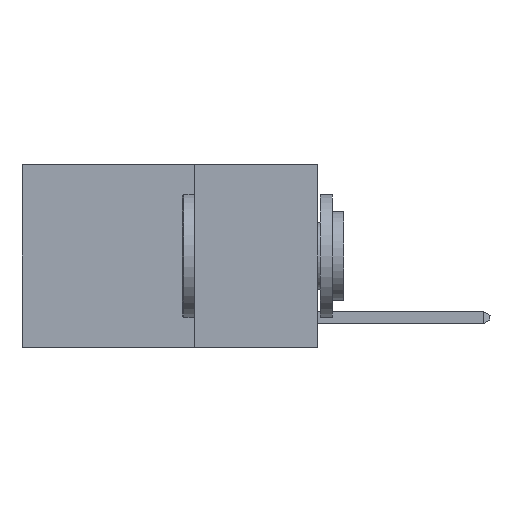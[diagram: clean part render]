
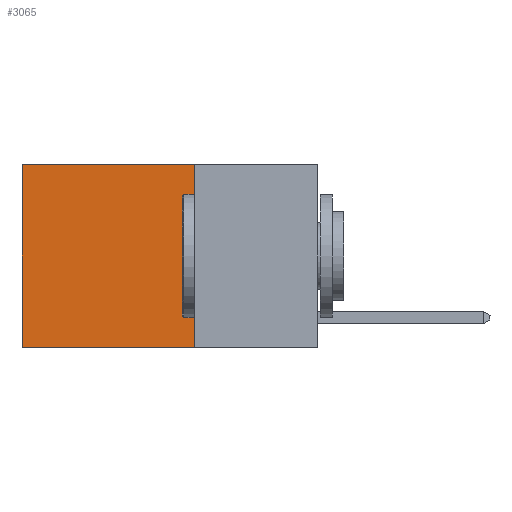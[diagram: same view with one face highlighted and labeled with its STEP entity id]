
A CAD part, left-side view. The second image highlights one B-rep face of the part: STEP entity #3065.
In plain terms, the highlighted planar face has unit normal (-1, 0, 0).
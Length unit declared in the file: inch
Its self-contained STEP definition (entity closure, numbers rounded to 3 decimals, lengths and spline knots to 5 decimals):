
#379 = LINE ( 'NONE', #10572, #13702 ) ;
#809 = CARTESIAN_POINT ( 'NONE',  ( 0.2625, 0.25, 0. ) ) ;
#1155 = LINE ( 'NONE', #1375, #1506 ) ;
#1322 = CARTESIAN_POINT ( 'NONE',  ( 0.2625, 0.6, -0.37 ) ) ;
#1352 = CARTESIAN_POINT ( 'NONE',  ( 0.2625, 0.6, 0. ) ) ;
#1375 = CARTESIAN_POINT ( 'NONE',  ( 0.2625, 0.25, 0. ) ) ;
#1506 = VECTOR ( 'NONE', #14447, 39.37008 ) ;
#1515 = DIRECTION ( 'NONE',  ( 1., 0., 0. ) ) ;
#1536 = EDGE_CURVE ( 'NONE', #3499, #5440, #1155, .T. ) ;
#2265 = EDGE_LOOP ( 'NONE', ( #4382, #9099, #7632, #3853 ) ) ;
#2464 = DIRECTION ( 'NONE',  ( 0., 0., -1. ) ) ;
#3065 = ADVANCED_FACE ( 'NONE', ( #7215 ), #10969, .F. ) ;
#3499 = VERTEX_POINT ( 'NONE', #809 ) ;
#3853 = ORIENTED_EDGE ( 'NONE', *, *, #1536, .T. ) ;
#4382 = ORIENTED_EDGE ( 'NONE', *, *, #10804, .T. ) ;
#5035 = AXIS2_PLACEMENT_3D ( 'NONE', #14340, #1515, #13237 ) ;
#5241 = VERTEX_POINT ( 'NONE', #8696 ) ;
#5434 = DIRECTION ( 'NONE',  ( 0., 0., -1. ) ) ;
#5440 = VERTEX_POINT ( 'NONE', #1352 ) ;
#5818 = VECTOR ( 'NONE', #9249, 39.37008 ) ;
#6788 = LINE ( 'NONE', #11366, #7745 ) ;
#7215 = FACE_OUTER_BOUND ( 'NONE', #2265, .T. ) ;
#7632 = ORIENTED_EDGE ( 'NONE', *, *, #13940, .F. ) ;
#7745 = VECTOR ( 'NONE', #5434, 39.37008 ) ;
#8114 = EDGE_CURVE ( 'NONE', #5241, #11723, #12476, .T. ) ;
#8696 = CARTESIAN_POINT ( 'NONE',  ( 0.2625, 0.25, -0.37 ) ) ;
#9099 = ORIENTED_EDGE ( 'NONE', *, *, #8114, .F. ) ;
#9249 = DIRECTION ( 'NONE',  ( 0., 1., 0. ) ) ;
#10572 = CARTESIAN_POINT ( 'NONE',  ( 0.2625, 0.6, 0. ) ) ;
#10804 = EDGE_CURVE ( 'NONE', #5440, #11723, #379, .T. ) ;
#10969 = PLANE ( 'NONE',  #5035 ) ;
#11366 = CARTESIAN_POINT ( 'NONE',  ( 0.2625, 0.25, 0. ) ) ;
#11723 = VERTEX_POINT ( 'NONE', #1322 ) ;
#12476 = LINE ( 'NONE', #13522, #5818 ) ;
#13237 = DIRECTION ( 'NONE',  ( 0., 0., -1. ) ) ;
#13522 = CARTESIAN_POINT ( 'NONE',  ( 0.2625, 0.25, -0.37 ) ) ;
#13702 = VECTOR ( 'NONE', #2464, 39.37008 ) ;
#13940 = EDGE_CURVE ( 'NONE', #3499, #5241, #6788, .T. ) ;
#14340 = CARTESIAN_POINT ( 'NONE',  ( 0.2625, 0.25, 0. ) ) ;
#14447 = DIRECTION ( 'NONE',  ( 0., 1., 0. ) ) ;
